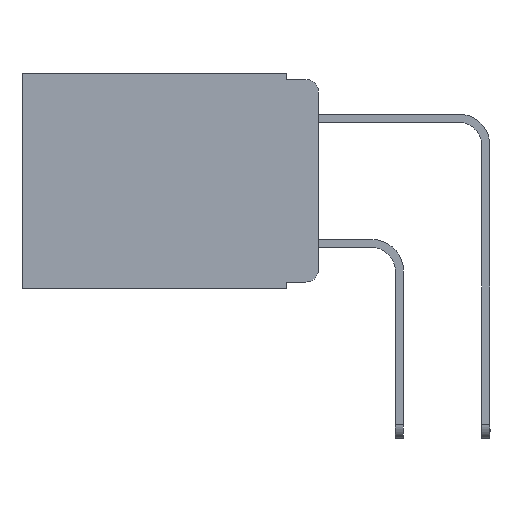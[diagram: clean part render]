
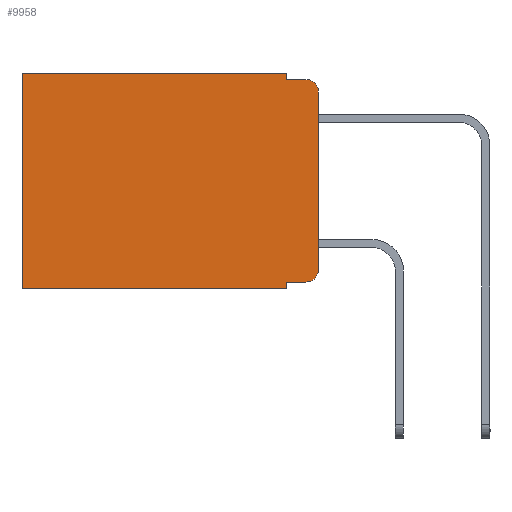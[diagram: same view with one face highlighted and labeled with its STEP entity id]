
A CAD part, left-side view. The second image highlights one B-rep face of the part: STEP entity #9958.
In plain terms, the highlighted planar face has unit normal (-1, 0, 0).
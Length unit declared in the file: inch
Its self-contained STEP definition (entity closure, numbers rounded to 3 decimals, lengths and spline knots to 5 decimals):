
#143 = VECTOR ( 'NONE', #9268, 39.37008 ) ;
#260 = CARTESIAN_POINT ( 'NONE',  ( 0.298, 0., -0.343 ) ) ;
#390 = LINE ( 'NONE', #7981, #9602 ) ;
#690 = LINE ( 'NONE', #19649, #143 ) ;
#1152 = ORIENTED_EDGE ( 'NONE', *, *, #17613, .T. ) ;
#1260 = CARTESIAN_POINT ( 'NONE',  ( 0.298, 0.051, -0.01 ) ) ;
#1478 = ORIENTED_EDGE ( 'NONE', *, *, #6126, .F. ) ;
#1510 = ORIENTED_EDGE ( 'NONE', *, *, #2266, .F. ) ;
#1679 = ORIENTED_EDGE ( 'NONE', *, *, #8216, .T. ) ;
#1696 = ORIENTED_EDGE ( 'NONE', *, *, #7432, .T. ) ;
#1732 = VERTEX_POINT ( 'NONE', #16170 ) ;
#2266 = EDGE_CURVE ( 'NONE', #17777, #17851, #690, .T. ) ;
#2421 = CARTESIAN_POINT ( 'NONE',  ( 0.298, 0.02, -0.03 ) ) ;
#2607 = AXIS2_PLACEMENT_3D ( 'NONE', #12660, #5805, #19824 ) ;
#2682 = DIRECTION ( 'NONE',  ( 0., 1., 0. ) ) ;
#2980 = VERTEX_POINT ( 'NONE', #13390 ) ;
#3060 = EDGE_CURVE ( 'NONE', #2980, #7067, #390, .T. ) ;
#3432 = ORIENTED_EDGE ( 'NONE', *, *, #3060, .T. ) ;
#3473 = CARTESIAN_POINT ( 'NONE',  ( 0.298, 0.051, 0. ) ) ;
#3650 = CARTESIAN_POINT ( 'NONE',  ( 0.298, 0.473, -0.343 ) ) ;
#4395 = EDGE_CURVE ( 'NONE', #9956, #7067, #22274, .T. ) ;
#5533 = CIRCLE ( 'NONE', #7224, 0.02 ) ;
#5805 = DIRECTION ( 'NONE',  ( 1., 0., 0. ) ) ;
#6126 = EDGE_CURVE ( 'NONE', #1732, #6404, #21660, .T. ) ;
#6202 = CARTESIAN_POINT ( 'NONE',  ( 0.298, 0.051, 0. ) ) ;
#6404 = VERTEX_POINT ( 'NONE', #10952 ) ;
#7018 = VECTOR ( 'NONE', #13216, 39.37008 ) ;
#7067 = VERTEX_POINT ( 'NONE', #3650 ) ;
#7224 = AXIS2_PLACEMENT_3D ( 'NONE', #2421, #14438, #14507 ) ;
#7371 = CARTESIAN_POINT ( 'NONE',  ( 0.298, 0.02, -0.333 ) ) ;
#7432 = EDGE_CURVE ( 'NONE', #17777, #2980, #16698, .T. ) ;
#7896 = VERTEX_POINT ( 'NONE', #22396 ) ;
#7981 = CARTESIAN_POINT ( 'NONE',  ( 0.298, 0.473, 0. ) ) ;
#8175 = ORIENTED_EDGE ( 'NONE', *, *, #4395, .F. ) ;
#8216 = EDGE_CURVE ( 'NONE', #18805, #21535, #11008, .T. ) ;
#8580 = VECTOR ( 'NONE', #2682, 39.37008 ) ;
#9175 = DIRECTION ( 'NONE',  ( 0., 0., -1. ) ) ;
#9268 = DIRECTION ( 'NONE',  ( 0., 0., -1. ) ) ;
#9341 = FACE_OUTER_BOUND ( 'NONE', #11158, .T. ) ;
#9602 = VECTOR ( 'NONE', #9723, 39.37008 ) ;
#9675 = DIRECTION ( 'NONE',  ( 0., -1., 0. ) ) ;
#9723 = DIRECTION ( 'NONE',  ( 0., 0., -1. ) ) ;
#9791 = ORIENTED_EDGE ( 'NONE', *, *, #13751, .F. ) ;
#9867 = CARTESIAN_POINT ( 'NONE',  ( 0.298, 0., 0. ) ) ;
#9956 = VERTEX_POINT ( 'NONE', #18067 ) ;
#9958 = ADVANCED_FACE ( 'NONE', ( #9341 ), #16454, .F. ) ;
#10399 = DIRECTION ( 'NONE',  ( 0., 0., -1. ) ) ;
#10413 = EDGE_CURVE ( 'NONE', #21535, #6404, #14145, .T. ) ;
#10462 = DIRECTION ( 'NONE',  ( 0., 1., 0. ) ) ;
#10952 = CARTESIAN_POINT ( 'NONE',  ( 0.298, 0., -0.313 ) ) ;
#11008 = LINE ( 'NONE', #16473, #12861 ) ;
#11158 = EDGE_LOOP ( 'NONE', ( #1478, #1152, #9791, #1510, #1696, #3432, #8175, #13693, #1679, #20418 ) ) ;
#11347 = CARTESIAN_POINT ( 'NONE',  ( 0.298, 0., 0. ) ) ;
#12561 = DIRECTION ( 'NONE',  ( -1., 0., 0. ) ) ;
#12660 = CARTESIAN_POINT ( 'NONE',  ( 0.298, 0., 0. ) ) ;
#12861 = VECTOR ( 'NONE', #9675, 39.37008 ) ;
#13216 = DIRECTION ( 'NONE',  ( 0., 0., -1. ) ) ;
#13390 = CARTESIAN_POINT ( 'NONE',  ( 0.298, 0.473, 0. ) ) ;
#13614 = AXIS2_PLACEMENT_3D ( 'NONE', #21088, #12561, #9175 ) ;
#13693 = ORIENTED_EDGE ( 'NONE', *, *, #20666, .F. ) ;
#13751 = EDGE_CURVE ( 'NONE', #17851, #7896, #14503, .T. ) ;
#14145 = CIRCLE ( 'NONE', #13614, 0.02 ) ;
#14438 = DIRECTION ( 'NONE',  ( -1., 0., 0. ) ) ;
#14503 = LINE ( 'NONE', #17531, #22407 ) ;
#14507 = DIRECTION ( 'NONE',  ( 0., 0., -1. ) ) ;
#16170 = CARTESIAN_POINT ( 'NONE',  ( 0.298, 0., -0.03 ) ) ;
#16454 = PLANE ( 'NONE',  #2607 ) ;
#16473 = CARTESIAN_POINT ( 'NONE',  ( 0.298, 0.051, -0.333 ) ) ;
#16698 = LINE ( 'NONE', #9867, #8580 ) ;
#17531 = CARTESIAN_POINT ( 'NONE',  ( 0.298, 0.051, -0.01 ) ) ;
#17613 = EDGE_CURVE ( 'NONE', #1732, #7896, #5533, .T. ) ;
#17777 = VERTEX_POINT ( 'NONE', #6202 ) ;
#17842 = LINE ( 'NONE', #3473, #21137 ) ;
#17851 = VERTEX_POINT ( 'NONE', #1260 ) ;
#18067 = CARTESIAN_POINT ( 'NONE',  ( 0.298, 0.051, -0.343 ) ) ;
#18219 = VECTOR ( 'NONE', #10462, 39.37008 ) ;
#18805 = VERTEX_POINT ( 'NONE', #21403 ) ;
#19279 = DIRECTION ( 'NONE',  ( 0., -1., 0. ) ) ;
#19649 = CARTESIAN_POINT ( 'NONE',  ( 0.298, 0.051, 0. ) ) ;
#19824 = DIRECTION ( 'NONE',  ( 0., 0., -1. ) ) ;
#20418 = ORIENTED_EDGE ( 'NONE', *, *, #10413, .T. ) ;
#20666 = EDGE_CURVE ( 'NONE', #18805, #9956, #17842, .T. ) ;
#21088 = CARTESIAN_POINT ( 'NONE',  ( 0.298, 0.02, -0.313 ) ) ;
#21137 = VECTOR ( 'NONE', #10399, 39.37008 ) ;
#21403 = CARTESIAN_POINT ( 'NONE',  ( 0.298, 0.051, -0.333 ) ) ;
#21535 = VERTEX_POINT ( 'NONE', #7371 ) ;
#21660 = LINE ( 'NONE', #11347, #7018 ) ;
#22274 = LINE ( 'NONE', #260, #18219 ) ;
#22396 = CARTESIAN_POINT ( 'NONE',  ( 0.298, 0.02, -0.01 ) ) ;
#22407 = VECTOR ( 'NONE', #19279, 39.37008 ) ;
